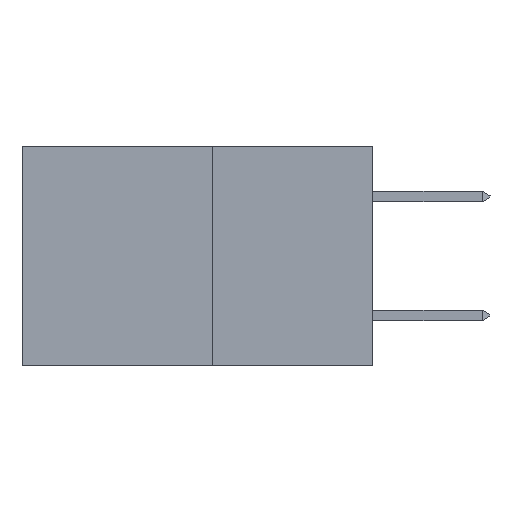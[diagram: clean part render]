
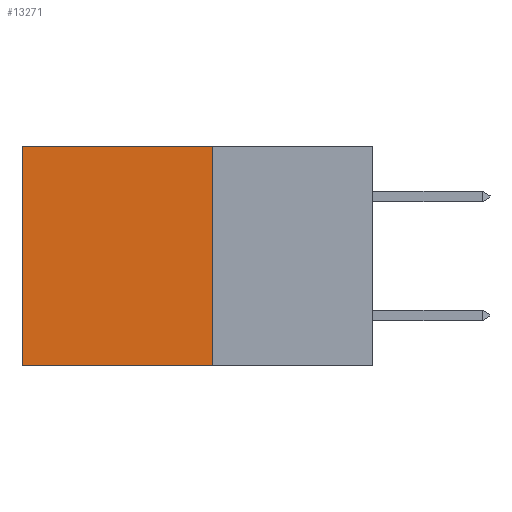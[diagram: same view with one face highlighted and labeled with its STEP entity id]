
A CAD part, left-side view. The second image highlights one B-rep face of the part: STEP entity #13271.
In plain terms, the highlighted planar face has unit normal (-1, 0, 0).
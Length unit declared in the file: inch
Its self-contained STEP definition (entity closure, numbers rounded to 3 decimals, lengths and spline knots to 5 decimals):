
#193 = DIRECTION ( 'NONE',  ( 0., 1., 0. ) ) ;
#578 = CARTESIAN_POINT ( 'NONE',  ( 0.277, 0.27, 0. ) ) ;
#1130 = LINE ( 'NONE', #28060, #15810 ) ;
#2050 = PLANE ( 'NONE',  #32782 ) ;
#2863 = VECTOR ( 'NONE', #193, 39.37008 ) ;
#3785 = VERTEX_POINT ( 'NONE', #578 ) ;
#4136 = DIRECTION ( 'NONE',  ( 0., 0., -1. ) ) ;
#4457 = DIRECTION ( 'NONE',  ( 0., 1., 0. ) ) ;
#4876 = DIRECTION ( 'NONE',  ( 0., 0., -1. ) ) ;
#4934 = VERTEX_POINT ( 'NONE', #29869 ) ;
#4940 = ORIENTED_EDGE ( 'NONE', *, *, #35314, .F. ) ;
#7074 = EDGE_CURVE ( 'NONE', #33505, #32612, #10248, .T. ) ;
#8355 = VECTOR ( 'NONE', #4136, 39.37008 ) ;
#8881 = EDGE_CURVE ( 'NONE', #3785, #4934, #22195, .T. ) ;
#8882 = ORIENTED_EDGE ( 'NONE', *, *, #30928, .T. ) ;
#9091 = FACE_OUTER_BOUND ( 'NONE', #30208, .T. ) ;
#10248 = LINE ( 'NONE', #24826, #2863 ) ;
#11679 = DIRECTION ( 'NONE',  ( 0., 0., -1. ) ) ;
#13022 = CARTESIAN_POINT ( 'NONE',  ( 0.277, 0.27, -0.37 ) ) ;
#13271 = ADVANCED_FACE ( 'NONE', ( #9091 ), #2050, .F. ) ;
#15810 = VECTOR ( 'NONE', #11679, 39.37008 ) ;
#20440 = CARTESIAN_POINT ( 'NONE',  ( 0.277, 0.27, -0.37 ) ) ;
#21338 = DIRECTION ( 'NONE',  ( 1., 0., 0. ) ) ;
#22195 = LINE ( 'NONE', #23805, #33221 ) ;
#23805 = CARTESIAN_POINT ( 'NONE',  ( 0.277, 0.27, 0. ) ) ;
#23837 = LINE ( 'NONE', #26094, #8355 ) ;
#24826 = CARTESIAN_POINT ( 'NONE',  ( 0.277, 0.27, -0.37 ) ) ;
#24887 = ORIENTED_EDGE ( 'NONE', *, *, #8881, .T. ) ;
#25249 = CARTESIAN_POINT ( 'NONE',  ( 0.277, 0.59, -0.37 ) ) ;
#26094 = CARTESIAN_POINT ( 'NONE',  ( 0.277, 0.59, -0.37 ) ) ;
#28060 = CARTESIAN_POINT ( 'NONE',  ( 0.277, 0.27, -0.37 ) ) ;
#29395 = ORIENTED_EDGE ( 'NONE', *, *, #7074, .F. ) ;
#29869 = CARTESIAN_POINT ( 'NONE',  ( 0.277, 0.59, 0. ) ) ;
#30208 = EDGE_LOOP ( 'NONE', ( #8882, #29395, #4940, #24887 ) ) ;
#30928 = EDGE_CURVE ( 'NONE', #4934, #32612, #23837, .T. ) ;
#32612 = VERTEX_POINT ( 'NONE', #25249 ) ;
#32782 = AXIS2_PLACEMENT_3D ( 'NONE', #13022, #21338, #4876 ) ;
#33221 = VECTOR ( 'NONE', #4457, 39.37008 ) ;
#33505 = VERTEX_POINT ( 'NONE', #20440 ) ;
#35314 = EDGE_CURVE ( 'NONE', #3785, #33505, #1130, .T. ) ;
